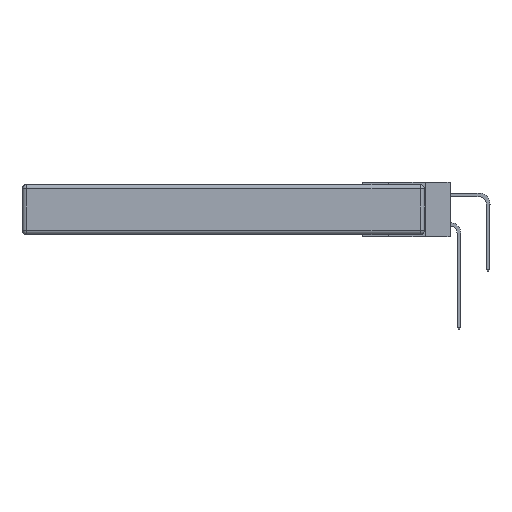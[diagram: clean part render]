
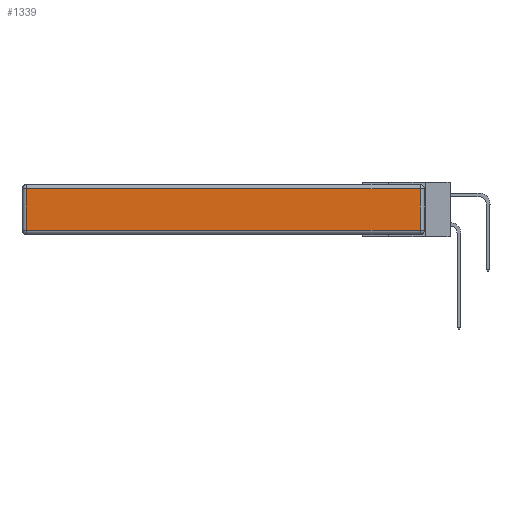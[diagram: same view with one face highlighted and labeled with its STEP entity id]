
A CAD part, left-side view. The second image highlights one B-rep face of the part: STEP entity #1339.
In plain terms, the highlighted planar face has unit normal (-1, 0, 0).
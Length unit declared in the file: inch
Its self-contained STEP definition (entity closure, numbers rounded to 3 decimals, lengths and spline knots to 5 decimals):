
#718 = ORIENTED_EDGE ( 'NONE', *, *, #29134, .T. ) ;
#808 = CARTESIAN_POINT ( 'NONE',  ( 0., 2.72, -0.343 ) ) ;
#1339 = ADVANCED_FACE ( 'NONE', ( #23414 ), #20651, .T. ) ;
#1516 = CARTESIAN_POINT ( 'NONE',  ( 0., 2.72, -0.03 ) ) ;
#2796 = CARTESIAN_POINT ( 'NONE',  ( 0., 2.72, -0.313 ) ) ;
#3357 = VERTEX_POINT ( 'NONE', #1516 ) ;
#3376 = LINE ( 'NONE', #808, #14802 ) ;
#3430 = EDGE_LOOP ( 'NONE', ( #5822, #14280, #718, #10533 ) ) ;
#4867 = CARTESIAN_POINT ( 'NONE',  ( 0., 0.03, -0.03 ) ) ;
#5822 = ORIENTED_EDGE ( 'NONE', *, *, #19281, .T. ) ;
#6085 = LINE ( 'NONE', #26680, #19953 ) ;
#6545 = LINE ( 'NONE', #20763, #15793 ) ;
#7155 = CARTESIAN_POINT ( 'NONE',  ( 0., 0., -0.343 ) ) ;
#7644 = DIRECTION ( 'NONE',  ( 0., 0., -1. ) ) ;
#8260 = DIRECTION ( 'NONE',  ( 0., 1., 0. ) ) ;
#8439 = DIRECTION ( 'NONE',  ( 0., 0., 1. ) ) ;
#9434 = DIRECTION ( 'NONE',  ( -1., 0., 0. ) ) ;
#9558 = VERTEX_POINT ( 'NONE', #2796 ) ;
#10391 = EDGE_CURVE ( 'NONE', #25992, #22146, #6085, .T. ) ;
#10533 = ORIENTED_EDGE ( 'NONE', *, *, #18359, .T. ) ;
#12263 = CARTESIAN_POINT ( 'NONE',  ( 0., 0.03, -0.313 ) ) ;
#13615 = VECTOR ( 'NONE', #8260, 39.37008 ) ;
#14280 = ORIENTED_EDGE ( 'NONE', *, *, #10391, .T. ) ;
#14802 = VECTOR ( 'NONE', #7644, 39.37008 ) ;
#15793 = VECTOR ( 'NONE', #20964, 39.37008 ) ;
#17546 = LINE ( 'NONE', #23879, #13615 ) ;
#18359 = EDGE_CURVE ( 'NONE', #3357, #9558, #3376, .T. ) ;
#19183 = AXIS2_PLACEMENT_3D ( 'NONE', #7155, #9434, #27588 ) ;
#19281 = EDGE_CURVE ( 'NONE', #9558, #25992, #6545, .T. ) ;
#19953 = VECTOR ( 'NONE', #8439, 39.37008 ) ;
#20651 = PLANE ( 'NONE',  #19183 ) ;
#20763 = CARTESIAN_POINT ( 'NONE',  ( 0., 0., -0.313 ) ) ;
#20964 = DIRECTION ( 'NONE',  ( 0., -1., 0. ) ) ;
#22146 = VERTEX_POINT ( 'NONE', #4867 ) ;
#23414 = FACE_OUTER_BOUND ( 'NONE', #3430, .T. ) ;
#23879 = CARTESIAN_POINT ( 'NONE',  ( 0., 2.75, -0.03 ) ) ;
#25992 = VERTEX_POINT ( 'NONE', #12263 ) ;
#26680 = CARTESIAN_POINT ( 'NONE',  ( 0., 0.03, -0.343 ) ) ;
#27588 = DIRECTION ( 'NONE',  ( 0., 0., 1. ) ) ;
#29134 = EDGE_CURVE ( 'NONE', #22146, #3357, #17546, .T. ) ;
